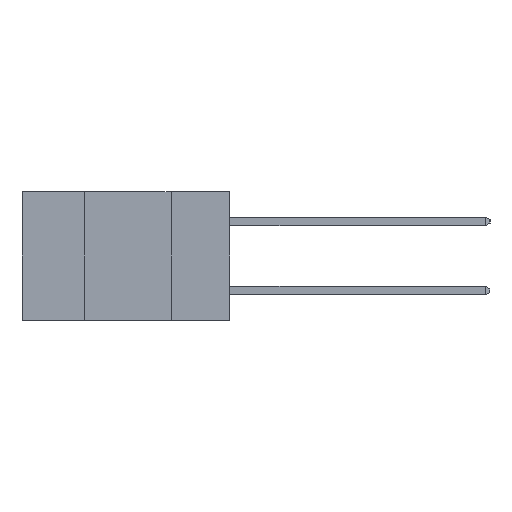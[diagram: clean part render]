
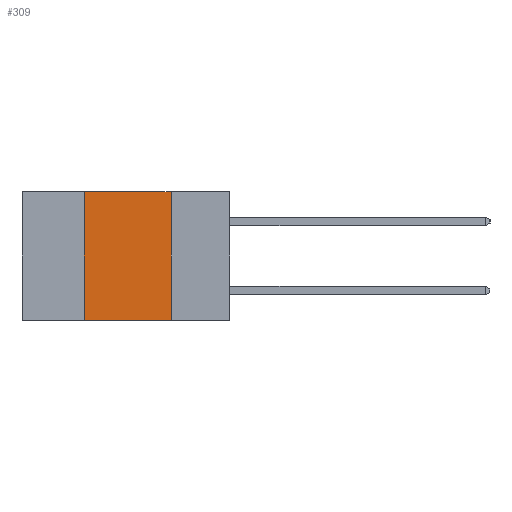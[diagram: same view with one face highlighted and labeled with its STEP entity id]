
A CAD part, left-side view. The second image highlights one B-rep face of the part: STEP entity #309.
In plain terms, the highlighted planar face has unit normal (-1, 0, 0).
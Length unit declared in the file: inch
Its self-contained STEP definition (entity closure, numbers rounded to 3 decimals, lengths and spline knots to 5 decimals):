
#309 = ADVANCED_FACE ( 'NONE', ( #10815 ), #3446, .F. ) ;
#804 = CARTESIAN_POINT ( 'NONE',  ( 0., 0.6, 0. ) ) ;
#1487 = VERTEX_POINT ( 'NONE', #17199 ) ;
#2174 = CARTESIAN_POINT ( 'NONE',  ( 0., 0.6, 0. ) ) ;
#2978 = ORIENTED_EDGE ( 'NONE', *, *, #7384, .F. ) ;
#3426 = DIRECTION ( 'NONE',  ( 1., 0., 0. ) ) ;
#3446 = PLANE ( 'NONE',  #8217 ) ;
#3549 = LINE ( 'NONE', #18266, #27893 ) ;
#3656 = EDGE_CURVE ( 'NONE', #1487, #19568, #9087, .T. ) ;
#7120 = VERTEX_POINT ( 'NONE', #25762 ) ;
#7384 = EDGE_CURVE ( 'NONE', #24922, #1487, #27336, .T. ) ;
#8217 = AXIS2_PLACEMENT_3D ( 'NONE', #2174, #3426, #30286 ) ;
#8507 = VECTOR ( 'NONE', #12543, 39.37008 ) ;
#9087 = LINE ( 'NONE', #24442, #20956 ) ;
#9957 = EDGE_CURVE ( 'NONE', #7120, #24922, #3549, .T. ) ;
#10571 = EDGE_CURVE ( 'NONE', #7120, #19568, #18694, .T. ) ;
#10815 = FACE_OUTER_BOUND ( 'NONE', #11922, .T. ) ;
#11691 = CARTESIAN_POINT ( 'NONE',  ( 0., 0.17, -0.37 ) ) ;
#11922 = EDGE_LOOP ( 'NONE', ( #15887, #2978, #28046, #17033 ) ) ;
#12543 = DIRECTION ( 'NONE',  ( 0., -1., 0. ) ) ;
#15887 = ORIENTED_EDGE ( 'NONE', *, *, #3656, .F. ) ;
#17033 = ORIENTED_EDGE ( 'NONE', *, *, #10571, .T. ) ;
#17199 = CARTESIAN_POINT ( 'NONE',  ( 0., 0.17, 0. ) ) ;
#18266 = CARTESIAN_POINT ( 'NONE',  ( 0., 0.42, 0. ) ) ;
#18694 = LINE ( 'NONE', #22571, #30417 ) ;
#19568 = VERTEX_POINT ( 'NONE', #11691 ) ;
#19780 = CARTESIAN_POINT ( 'NONE',  ( 0., 0.42, 0. ) ) ;
#20173 = DIRECTION ( 'NONE',  ( 0., -1., 0. ) ) ;
#20613 = DIRECTION ( 'NONE',  ( 0., 0., 1. ) ) ;
#20956 = VECTOR ( 'NONE', #26795, 39.37008 ) ;
#22571 = CARTESIAN_POINT ( 'NONE',  ( 0., 0.6, -0.37 ) ) ;
#24442 = CARTESIAN_POINT ( 'NONE',  ( 0., 0.17, 0. ) ) ;
#24922 = VERTEX_POINT ( 'NONE', #19780 ) ;
#25762 = CARTESIAN_POINT ( 'NONE',  ( 0., 0.42, -0.37 ) ) ;
#26795 = DIRECTION ( 'NONE',  ( 0., 0., -1. ) ) ;
#27336 = LINE ( 'NONE', #804, #8507 ) ;
#27893 = VECTOR ( 'NONE', #20613, 39.37008 ) ;
#28046 = ORIENTED_EDGE ( 'NONE', *, *, #9957, .F. ) ;
#30286 = DIRECTION ( 'NONE',  ( 0., 0., -1. ) ) ;
#30417 = VECTOR ( 'NONE', #20173, 39.37008 ) ;
